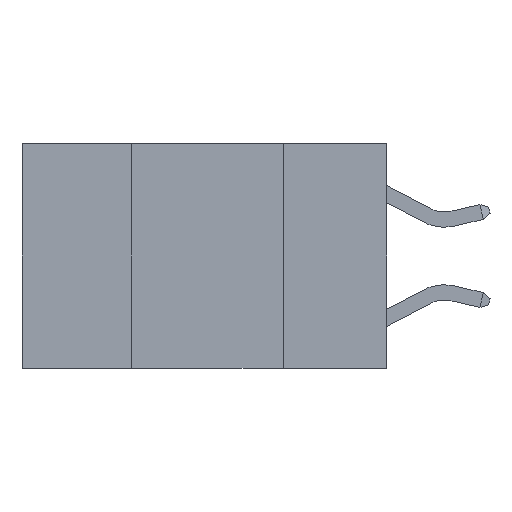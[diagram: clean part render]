
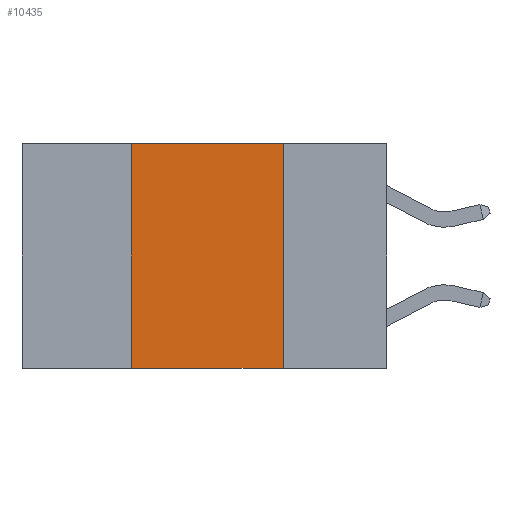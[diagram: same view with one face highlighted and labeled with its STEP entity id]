
A CAD part, left-side view. The second image highlights one B-rep face of the part: STEP entity #10435.
In plain terms, the highlighted planar face has unit normal (-1, 0, 0).
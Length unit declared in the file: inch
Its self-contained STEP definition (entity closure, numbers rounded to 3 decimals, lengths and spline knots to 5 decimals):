
#29 = CARTESIAN_POINT ( 'NONE',  ( 0., 0.17, 0. ) ) ;
#717 = CARTESIAN_POINT ( 'NONE',  ( 0., 0.42, 0. ) ) ;
#1529 = LINE ( 'NONE', #8394, #16247 ) ;
#2474 = AXIS2_PLACEMENT_3D ( 'NONE', #15171, #13475, #20330 ) ;
#2669 = CARTESIAN_POINT ( 'NONE',  ( 0., 0.17, 0. ) ) ;
#3866 = CARTESIAN_POINT ( 'NONE',  ( 0., 0.6, 0. ) ) ;
#4185 = VERTEX_POINT ( 'NONE', #11824 ) ;
#4236 = DIRECTION ( 'NONE',  ( 0., 0., -1. ) ) ;
#4272 = VECTOR ( 'NONE', #7708, 39.37008 ) ;
#4665 = ORIENTED_EDGE ( 'NONE', *, *, #13876, .F. ) ;
#5740 = ORIENTED_EDGE ( 'NONE', *, *, #14032, .T. ) ;
#5850 = ORIENTED_EDGE ( 'NONE', *, *, #6602, .F. ) ;
#5863 = CARTESIAN_POINT ( 'NONE',  ( 0., 0.42, 0. ) ) ;
#6496 = PLANE ( 'NONE',  #2474 ) ;
#6602 = EDGE_CURVE ( 'NONE', #4185, #17001, #14252, .T. ) ;
#7708 = DIRECTION ( 'NONE',  ( 0., -1., 0. ) ) ;
#8394 = CARTESIAN_POINT ( 'NONE',  ( 0., 0.6, -0.37 ) ) ;
#9976 = DIRECTION ( 'NONE',  ( 0., -1., 0. ) ) ;
#10132 = VECTOR ( 'NONE', #4236, 39.37008 ) ;
#10435 = ADVANCED_FACE ( 'NONE', ( #21918 ), #6496, .F. ) ;
#10712 = EDGE_CURVE ( 'NONE', #17001, #16481, #16278, .T. ) ;
#11759 = VERTEX_POINT ( 'NONE', #20840 ) ;
#11824 = CARTESIAN_POINT ( 'NONE',  ( 0., 0.42, -0.37 ) ) ;
#13204 = VECTOR ( 'NONE', #19539, 39.37008 ) ;
#13475 = DIRECTION ( 'NONE',  ( 1., 0., 0. ) ) ;
#13876 = EDGE_CURVE ( 'NONE', #16481, #11759, #18093, .T. ) ;
#14032 = EDGE_CURVE ( 'NONE', #4185, #11759, #1529, .T. ) ;
#14252 = LINE ( 'NONE', #717, #13204 ) ;
#14804 = EDGE_LOOP ( 'NONE', ( #4665, #15220, #5850, #5740 ) ) ;
#15171 = CARTESIAN_POINT ( 'NONE',  ( 0., 0.6, 0. ) ) ;
#15220 = ORIENTED_EDGE ( 'NONE', *, *, #10712, .F. ) ;
#16247 = VECTOR ( 'NONE', #9976, 39.37008 ) ;
#16278 = LINE ( 'NONE', #3866, #4272 ) ;
#16481 = VERTEX_POINT ( 'NONE', #29 ) ;
#17001 = VERTEX_POINT ( 'NONE', #5863 ) ;
#18093 = LINE ( 'NONE', #2669, #10132 ) ;
#19539 = DIRECTION ( 'NONE',  ( 0., 0., 1. ) ) ;
#20330 = DIRECTION ( 'NONE',  ( 0., 0., -1. ) ) ;
#20840 = CARTESIAN_POINT ( 'NONE',  ( 0., 0.17, -0.37 ) ) ;
#21918 = FACE_OUTER_BOUND ( 'NONE', #14804, .T. ) ;
